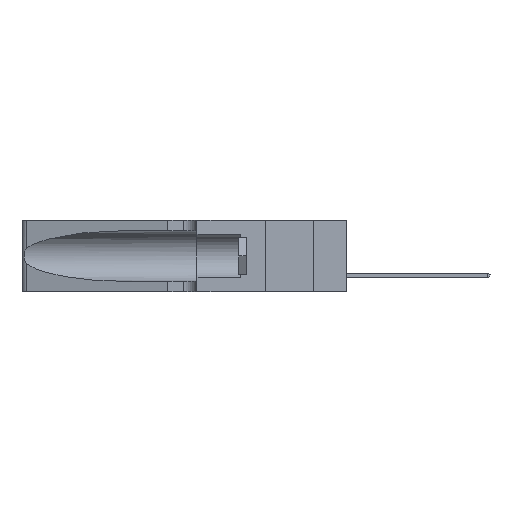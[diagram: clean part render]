
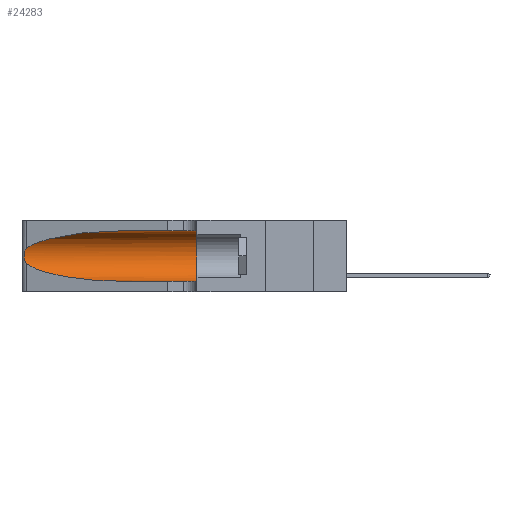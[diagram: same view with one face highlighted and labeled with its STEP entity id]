
A CAD part, left-side view. The second image highlights one B-rep face of the part: STEP entity #24283.
In plain terms, the highlighted cylindrical face has radius 3.308 mm (diameter 6.617 mm), a partial arc.
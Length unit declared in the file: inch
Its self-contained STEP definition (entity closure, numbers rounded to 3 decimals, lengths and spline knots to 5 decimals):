
#382 = CIRCLE ( 'NONE', #21893, 0.13025 ) ;
#726 = CARTESIAN_POINT ( 'NONE',  ( 0.1305, 0.72297, 0.31525 ) ) ;
#856 = CARTESIAN_POINT ( 'NONE',  ( 0.1305, 0.72297, 0.05475 ) ) ;
#1522 = EDGE_CURVE ( 'NONE', #22628, #24362, #10979, .T. ) ;
#1617 = CARTESIAN_POINT ( 'NONE',  ( 0.25487, 1.22718, 0.14631 ) ) ;
#2203 = CARTESIAN_POINT ( 'NONE',  ( 0.25487, 1.22718, 0.22369 ) ) ;
#2779 = VERTEX_POINT ( 'NONE', #14135 ) ;
#2836 =( BOUNDED_CURVE ( )  B_SPLINE_CURVE ( 3, ( #1617, #30320, #4817, #24747 ),
 .UNSPECIFIED., .F., .T. ) 
 B_SPLINE_CURVE_WITH_KNOTS ( ( 4, 4 ),
 ( 3.44316, 4.71239 ),
 .UNSPECIFIED. ) 
 CURVE ( )  GEOMETRIC_REPRESENTATION_ITEM ( )  RATIONAL_B_SPLINE_CURVE ( ( 1., 0.87, 0.87, 1. ) ) 
 REPRESENTATION_ITEM ( '' )  );
#2879 = CARTESIAN_POINT ( 'NONE',  ( 0.25487, 1.22718, 0.22369 ) ) ;
#3466 = CARTESIAN_POINT ( 'NONE',  ( 0.1305, 1.61858, 0.185 ) ) ;
#3827 = CARTESIAN_POINT ( 'NONE',  ( 0.26018, 1.23835, 0.19895 ) ) ;
#3858 = CARTESIAN_POINT ( 'NONE',  ( 0.25487, 1.22718, 0.22369 ) ) ;
#4817 = CARTESIAN_POINT ( 'NONE',  ( 0.18966, 0.96281, 0.05475 ) ) ;
#6316 = DIRECTION ( 'NONE',  ( 0., -1., 0. ) ) ;
#6943 = CARTESIAN_POINT ( 'NONE',  ( 0.25787, 1.23484, 0.2124 ) ) ;
#9363 = EDGE_LOOP ( 'NONE', ( #33140, #21830, #16279, #28395, #23017, #13297 ) ) ;
#9532 = DIRECTION ( 'NONE',  ( 0., 0., -1. ) ) ;
#9796 = CARTESIAN_POINT ( 'NONE',  ( 0.25856, 1.23593, 0.16098 ) ) ;
#10979 = LINE ( 'NONE', #17076, #36341 ) ;
#11159 = DIRECTION ( 'NONE',  ( 0., -1., 0. ) ) ;
#11209 = B_SPLINE_CURVE_WITH_KNOTS ( 'NONE', 3,
 ( #2879, #30848, #30976, #6943, #26824, #3827, #15280, #23843, #12228, #9796, #29692, #24112, #12481, #26704 ),
 .UNSPECIFIED., .F., .F.,
 ( 4, 2, 2, 2, 2, 2, 4 ),
 ( 0., 0.00027, 0.00053, 0.00107, 0.0016, 0.00187, 0.00214 ),
 .UNSPECIFIED. ) ;
#12228 = CARTESIAN_POINT ( 'NONE',  ( 0.26017, 1.23833, 0.17102 ) ) ;
#12481 = CARTESIAN_POINT ( 'NONE',  ( 0.25555, 1.22993, 0.14849 ) ) ;
#13297 = ORIENTED_EDGE ( 'NONE', *, *, #1522, .F. ) ;
#13804 = DIRECTION ( 'NONE',  ( 0., 1., 0. ) ) ;
#14135 = CARTESIAN_POINT ( 'NONE',  ( 0.1305, 0.35, 0.05475 ) ) ;
#14496 = EDGE_CURVE ( 'NONE', #30528, #32684, #11209, .T. ) ;
#14523 = CARTESIAN_POINT ( 'NONE',  ( 0.1305, 0.72297, 0.31525 ) ) ;
#14792 = CARTESIAN_POINT ( 'NONE',  ( 0.18966, 0.96281, 0.31525 ) ) ;
#15280 = CARTESIAN_POINT ( 'NONE',  ( 0.26075, 1.23896, 0.19203 ) ) ;
#16279 = ORIENTED_EDGE ( 'NONE', *, *, #30048, .T. ) ;
#17076 = CARTESIAN_POINT ( 'NONE',  ( 0.1305, 1.61858, 0.31525 ) ) ;
#17821 = CARTESIAN_POINT ( 'NONE',  ( 0.2373, 1.15595, 0.28018 ) ) ;
#18137 = VECTOR ( 'NONE', #23754, 39.37008 ) ;
#18214 = FACE_OUTER_BOUND ( 'NONE', #9363, .T. ) ;
#18937 = EDGE_CURVE ( 'NONE', #24362, #2779, #382, .T. ) ;
#19702 = DIRECTION ( 'NONE',  ( 0., 0., 1. ) ) ;
#20392 = EDGE_CURVE ( 'NONE', #23735, #2779, #36755, .T. ) ;
#21830 = ORIENTED_EDGE ( 'NONE', *, *, #14496, .T. ) ;
#21893 = AXIS2_PLACEMENT_3D ( 'NONE', #26485, #13804, #19702 ) ;
#22628 = VERTEX_POINT ( 'NONE', #14523 ) ;
#23017 = ORIENTED_EDGE ( 'NONE', *, *, #18937, .F. ) ;
#23735 = VERTEX_POINT ( 'NONE', #856 ) ;
#23754 = DIRECTION ( 'NONE',  ( 0., -1., 0. ) ) ;
#23843 = CARTESIAN_POINT ( 'NONE',  ( 0.26075, 1.23896, 0.178 ) ) ;
#24112 = CARTESIAN_POINT ( 'NONE',  ( 0.25639, 1.23186, 0.15144 ) ) ;
#24257 = CARTESIAN_POINT ( 'NONE',  ( 0.25487, 1.22718, 0.14631 ) ) ;
#24283 = ADVANCED_FACE ( 'NONE', ( #18214 ), #31486, .F. ) ;
#24362 = VERTEX_POINT ( 'NONE', #33949 ) ;
#24747 = CARTESIAN_POINT ( 'NONE',  ( 0.1305, 0.72297, 0.05475 ) ) ;
#26332 = EDGE_CURVE ( 'NONE', #22628, #30528, #35850, .T. ) ;
#26485 = CARTESIAN_POINT ( 'NONE',  ( 0.1305, 0.35, 0.185 ) ) ;
#26704 = CARTESIAN_POINT ( 'NONE',  ( 0.25487, 1.22718, 0.14631 ) ) ;
#26824 = CARTESIAN_POINT ( 'NONE',  ( 0.25854, 1.2359, 0.20912 ) ) ;
#28395 = ORIENTED_EDGE ( 'NONE', *, *, #20392, .T. ) ;
#29692 = CARTESIAN_POINT ( 'NONE',  ( 0.25789, 1.23486, 0.15765 ) ) ;
#30048 = EDGE_CURVE ( 'NONE', #32684, #23735, #2836, .T. ) ;
#30320 = CARTESIAN_POINT ( 'NONE',  ( 0.2373, 1.15595, 0.08982 ) ) ;
#30528 = VERTEX_POINT ( 'NONE', #2203 ) ;
#30848 = CARTESIAN_POINT ( 'NONE',  ( 0.25555, 1.22994, 0.2215 ) ) ;
#30976 = CARTESIAN_POINT ( 'NONE',  ( 0.25639, 1.23184, 0.21858 ) ) ;
#31486 = CYLINDRICAL_SURFACE ( 'NONE', #32202, 0.13025 ) ;
#32078 = CARTESIAN_POINT ( 'NONE',  ( 0.1305, 1.61858, 0.05475 ) ) ;
#32202 = AXIS2_PLACEMENT_3D ( 'NONE', #3466, #6316, #9532 ) ;
#32684 = VERTEX_POINT ( 'NONE', #24257 ) ;
#33140 = ORIENTED_EDGE ( 'NONE', *, *, #26332, .T. ) ;
#33949 = CARTESIAN_POINT ( 'NONE',  ( 0.1305, 0.35, 0.31525 ) ) ;
#35850 =( BOUNDED_CURVE ( )  B_SPLINE_CURVE ( 3, ( #726, #14792, #17821, #3858 ),
 .UNSPECIFIED., .F., .T. ) 
 B_SPLINE_CURVE_WITH_KNOTS ( ( 4, 4 ),
 ( 1.5708, 2.84003 ),
 .UNSPECIFIED. ) 
 CURVE ( )  GEOMETRIC_REPRESENTATION_ITEM ( )  RATIONAL_B_SPLINE_CURVE ( ( 1., 0.87, 0.87, 1. ) ) 
 REPRESENTATION_ITEM ( '' )  );
#36341 = VECTOR ( 'NONE', #11159, 39.37008 ) ;
#36755 = LINE ( 'NONE', #32078, #18137 ) ;
